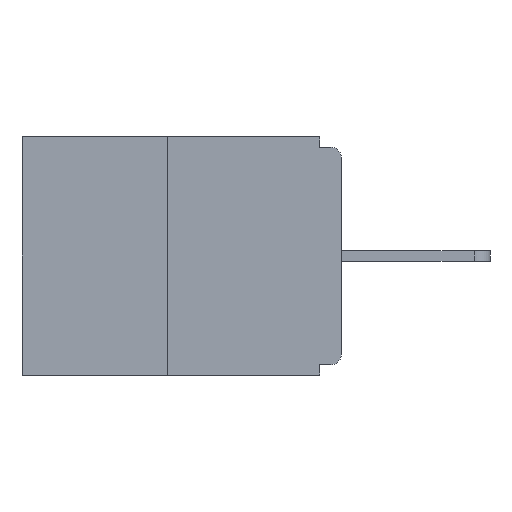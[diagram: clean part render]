
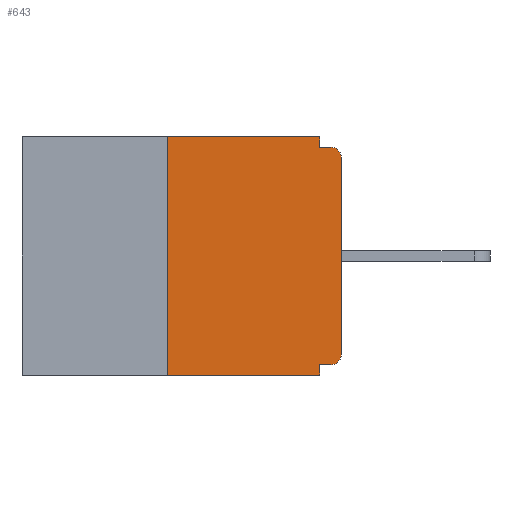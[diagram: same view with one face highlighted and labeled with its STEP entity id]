
A CAD part, left-side view. The second image highlights one B-rep face of the part: STEP entity #643.
In plain terms, the highlighted planar face has unit normal (-1, 0, 0).
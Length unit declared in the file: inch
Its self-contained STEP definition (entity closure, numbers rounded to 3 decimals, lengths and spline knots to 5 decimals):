
#64 = ORIENTED_EDGE ( 'NONE', *, *, #9942, .T. ) ;
#158 = ORIENTED_EDGE ( 'NONE', *, *, #8819, .T. ) ;
#169 = VERTEX_POINT ( 'NONE', #3978 ) ;
#260 = DIRECTION ( 'NONE',  ( -1., 0., 0. ) ) ;
#428 = CARTESIAN_POINT ( 'NONE',  ( 0., 0.015, -0.015 ) ) ;
#492 = ORIENTED_EDGE ( 'NONE', *, *, #995, .F. ) ;
#643 = ADVANCED_FACE ( 'NONE', ( #7188 ), #3114, .F. ) ;
#665 = VERTEX_POINT ( 'NONE', #8913 ) ;
#995 = EDGE_CURVE ( 'NONE', #4294, #5598, #5268, .T. ) ;
#1087 = VECTOR ( 'NONE', #8924, 39.37008 ) ;
#1299 = LINE ( 'NONE', #2950, #5522 ) ;
#1301 = DIRECTION ( 'NONE',  ( 0., 0., -1. ) ) ;
#1346 = ORIENTED_EDGE ( 'NONE', *, *, #1728, .T. ) ;
#1437 = VECTOR ( 'NONE', #7637, 39.37008 ) ;
#1496 = EDGE_CURVE ( 'NONE', #5598, #665, #8976, .T. ) ;
#1576 = CARTESIAN_POINT ( 'NONE',  ( 0., 0., -0.328 ) ) ;
#1728 = EDGE_CURVE ( 'NONE', #7347, #4047, #6465, .T. ) ;
#1762 = EDGE_CURVE ( 'NONE', #169, #4182, #10157, .T. ) ;
#1824 = EDGE_LOOP ( 'NONE', ( #3271, #492, #64, #5300, #9610, #1346, #2698, #158, #1978, #7142 ) ) ;
#1930 = EDGE_CURVE ( 'NONE', #6979, #9101, #6381, .T. ) ;
#1978 = ORIENTED_EDGE ( 'NONE', *, *, #1930, .F. ) ;
#1989 = CARTESIAN_POINT ( 'NONE',  ( 0., 0.015, -0.313 ) ) ;
#2001 = VECTOR ( 'NONE', #2328, 39.37008 ) ;
#2328 = DIRECTION ( 'NONE',  ( 0., -1., 0. ) ) ;
#2698 = ORIENTED_EDGE ( 'NONE', *, *, #9123, .T. ) ;
#2868 = CARTESIAN_POINT ( 'NONE',  ( 0., 0.46, -0.343 ) ) ;
#2950 = CARTESIAN_POINT ( 'NONE',  ( 0., 0., 0. ) ) ;
#2972 = CARTESIAN_POINT ( 'NONE',  ( 0., 0.25, -0.343 ) ) ;
#3114 = PLANE ( 'NONE',  #5404 ) ;
#3228 = LINE ( 'NONE', #1576, #1087 ) ;
#3271 = ORIENTED_EDGE ( 'NONE', *, *, #1496, .F. ) ;
#3524 = LINE ( 'NONE', #5292, #4831 ) ;
#3837 = DIRECTION ( 'NONE',  ( 0., 0., 1. ) ) ;
#3960 = CARTESIAN_POINT ( 'NONE',  ( 0., 0., -0.313 ) ) ;
#3978 = CARTESIAN_POINT ( 'NONE',  ( 0., 0.031, -0.328 ) ) ;
#4047 = VERTEX_POINT ( 'NONE', #3960 ) ;
#4182 = VERTEX_POINT ( 'NONE', #7384 ) ;
#4294 = VERTEX_POINT ( 'NONE', #2972 ) ;
#4412 = LINE ( 'NONE', #2868, #1437 ) ;
#4439 = DIRECTION ( 'NONE',  ( 0., 0., 1. ) ) ;
#4606 = DIRECTION ( 'NONE',  ( 1., 0., 0. ) ) ;
#4767 = CARTESIAN_POINT ( 'NONE',  ( 0., 0.46, 0. ) ) ;
#4831 = VECTOR ( 'NONE', #7776, 39.37008 ) ;
#4891 = VECTOR ( 'NONE', #3837, 39.37008 ) ;
#5155 = CARTESIAN_POINT ( 'NONE',  ( 0., 0.25, 0. ) ) ;
#5268 = LINE ( 'NONE', #7916, #4891 ) ;
#5292 = CARTESIAN_POINT ( 'NONE',  ( 0., 0.031, 0. ) ) ;
#5300 = ORIENTED_EDGE ( 'NONE', *, *, #1762, .F. ) ;
#5303 = DIRECTION ( 'NONE',  ( -1., 0., 0. ) ) ;
#5404 = AXIS2_PLACEMENT_3D ( 'NONE', #4767, #4606, #9672 ) ;
#5481 = CARTESIAN_POINT ( 'NONE',  ( 0., 0.46, 0. ) ) ;
#5522 = VECTOR ( 'NONE', #4439, 39.37008 ) ;
#5598 = VERTEX_POINT ( 'NONE', #5155 ) ;
#5713 = AXIS2_PLACEMENT_3D ( 'NONE', #9630, #5303, #8592 ) ;
#5829 = VERTEX_POINT ( 'NONE', #8140 ) ;
#6214 = DIRECTION ( 'NONE',  ( 0., 0., -1. ) ) ;
#6238 = CARTESIAN_POINT ( 'NONE',  ( 0., 0.015, -0.328 ) ) ;
#6381 = LINE ( 'NONE', #8057, #7148 ) ;
#6418 = EDGE_CURVE ( 'NONE', #665, #6979, #3524, .T. ) ;
#6465 = CIRCLE ( 'NONE', #10614, 0.015 ) ;
#6979 = VERTEX_POINT ( 'NONE', #8784 ) ;
#7142 = ORIENTED_EDGE ( 'NONE', *, *, #6418, .F. ) ;
#7148 = VECTOR ( 'NONE', #9884, 39.37008 ) ;
#7188 = FACE_OUTER_BOUND ( 'NONE', #1824, .T. ) ;
#7347 = VERTEX_POINT ( 'NONE', #6238 ) ;
#7384 = CARTESIAN_POINT ( 'NONE',  ( 0., 0.031, -0.343 ) ) ;
#7637 = DIRECTION ( 'NONE',  ( 0., -1., 0. ) ) ;
#7776 = DIRECTION ( 'NONE',  ( 0., 0., -1. ) ) ;
#7916 = CARTESIAN_POINT ( 'NONE',  ( 0., 0.25, 0. ) ) ;
#8057 = CARTESIAN_POINT ( 'NONE',  ( 0., 0., -0.015 ) ) ;
#8140 = CARTESIAN_POINT ( 'NONE',  ( 0., 0., -0.03 ) ) ;
#8533 = CARTESIAN_POINT ( 'NONE',  ( 0., 0.031, -0.343 ) ) ;
#8592 = DIRECTION ( 'NONE',  ( 0., 0., -1. ) ) ;
#8696 = VECTOR ( 'NONE', #1301, 39.37008 ) ;
#8784 = CARTESIAN_POINT ( 'NONE',  ( 0., 0.031, -0.015 ) ) ;
#8819 = EDGE_CURVE ( 'NONE', #5829, #9101, #10015, .T. ) ;
#8835 = EDGE_CURVE ( 'NONE', #7347, #169, #3228, .T. ) ;
#8913 = CARTESIAN_POINT ( 'NONE',  ( 0., 0.031, 0. ) ) ;
#8924 = DIRECTION ( 'NONE',  ( 0., 1., 0. ) ) ;
#8976 = LINE ( 'NONE', #5481, #2001 ) ;
#9101 = VERTEX_POINT ( 'NONE', #428 ) ;
#9123 = EDGE_CURVE ( 'NONE', #4047, #5829, #1299, .T. ) ;
#9610 = ORIENTED_EDGE ( 'NONE', *, *, #8835, .F. ) ;
#9630 = CARTESIAN_POINT ( 'NONE',  ( 0., 0.015, -0.03 ) ) ;
#9672 = DIRECTION ( 'NONE',  ( 0., 0., -1. ) ) ;
#9884 = DIRECTION ( 'NONE',  ( 0., -1., 0. ) ) ;
#9942 = EDGE_CURVE ( 'NONE', #4294, #4182, #4412, .T. ) ;
#10015 = CIRCLE ( 'NONE', #5713, 0.015 ) ;
#10157 = LINE ( 'NONE', #8533, #8696 ) ;
#10614 = AXIS2_PLACEMENT_3D ( 'NONE', #1989, #260, #6214 ) ;
